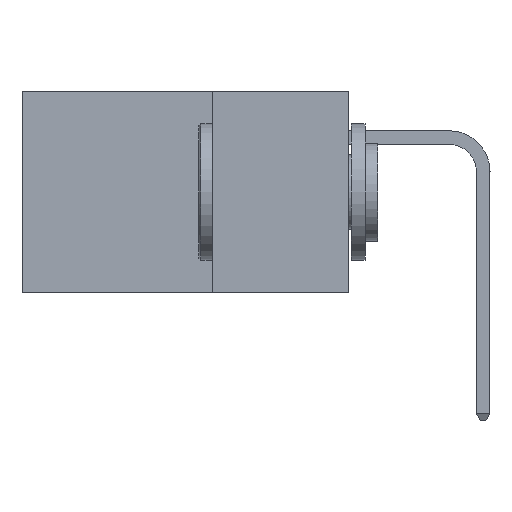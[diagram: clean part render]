
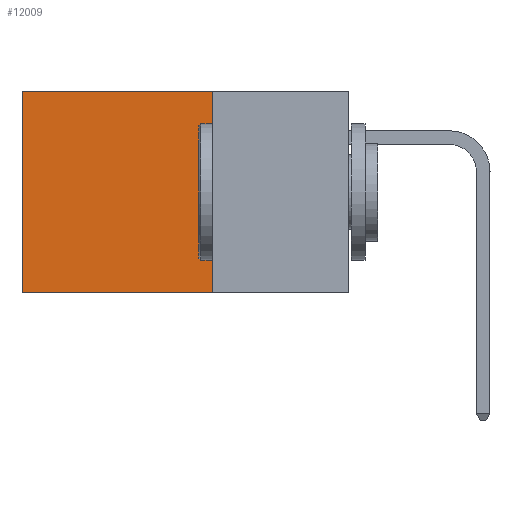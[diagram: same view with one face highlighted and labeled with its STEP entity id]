
A CAD part, left-side view. The second image highlights one B-rep face of the part: STEP entity #12009.
In plain terms, the highlighted planar face has unit normal (-1, 0, 0).
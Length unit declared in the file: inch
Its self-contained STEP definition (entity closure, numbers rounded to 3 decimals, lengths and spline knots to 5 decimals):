
#144 = PLANE ( 'NONE',  #20492 ) ;
#1122 = CARTESIAN_POINT ( 'NONE',  ( 0.2875, 0.6, 0. ) ) ;
#1136 = LINE ( 'NONE', #16714, #17392 ) ;
#1546 = VERTEX_POINT ( 'NONE', #5032 ) ;
#2478 = CARTESIAN_POINT ( 'NONE',  ( 0.2875, 0.25, 0. ) ) ;
#2580 = EDGE_CURVE ( 'NONE', #22776, #1546, #17502, .T. ) ;
#2743 = DIRECTION ( 'NONE',  ( 0., 0., -1. ) ) ;
#3334 = VECTOR ( 'NONE', #19300, 39.37008 ) ;
#3573 = CARTESIAN_POINT ( 'NONE',  ( 0.2875, 0.6, -0.37 ) ) ;
#3622 = VERTEX_POINT ( 'NONE', #3573 ) ;
#5032 = CARTESIAN_POINT ( 'NONE',  ( 0.2875, 0.6, 0. ) ) ;
#7667 = LINE ( 'NONE', #15661, #23456 ) ;
#8978 = CARTESIAN_POINT ( 'NONE',  ( 0.2875, 0.25, 0. ) ) ;
#9780 = ORIENTED_EDGE ( 'NONE', *, *, #13392, .F. ) ;
#12009 = ADVANCED_FACE ( 'NONE', ( #12944 ), #144, .F. ) ;
#12671 = VECTOR ( 'NONE', #15563, 39.37008 ) ;
#12944 = FACE_OUTER_BOUND ( 'NONE', #19693, .T. ) ;
#13011 = CARTESIAN_POINT ( 'NONE',  ( 0.2875, 0.25, 0. ) ) ;
#13283 = CARTESIAN_POINT ( 'NONE',  ( 0.2875, 0.25, -0.37 ) ) ;
#13392 = EDGE_CURVE ( 'NONE', #13552, #3622, #1136, .T. ) ;
#13552 = VERTEX_POINT ( 'NONE', #13283 ) ;
#13673 = EDGE_CURVE ( 'NONE', #22776, #13552, #7667, .T. ) ;
#14781 = ORIENTED_EDGE ( 'NONE', *, *, #16775, .T. ) ;
#15563 = DIRECTION ( 'NONE',  ( 0., 1., 0. ) ) ;
#15661 = CARTESIAN_POINT ( 'NONE',  ( 0.2875, 0.25, 0. ) ) ;
#16714 = CARTESIAN_POINT ( 'NONE',  ( 0.2875, 0.25, -0.37 ) ) ;
#16775 = EDGE_CURVE ( 'NONE', #1546, #3622, #23654, .T. ) ;
#17392 = VECTOR ( 'NONE', #20325, 39.37008 ) ;
#17502 = LINE ( 'NONE', #2478, #12671 ) ;
#17533 = ORIENTED_EDGE ( 'NONE', *, *, #2580, .T. ) ;
#17984 = DIRECTION ( 'NONE',  ( 0., 0., -1. ) ) ;
#18344 = DIRECTION ( 'NONE',  ( 1., 0., 0. ) ) ;
#19300 = DIRECTION ( 'NONE',  ( 0., 0., -1. ) ) ;
#19693 = EDGE_LOOP ( 'NONE', ( #14781, #9780, #20884, #17533 ) ) ;
#20325 = DIRECTION ( 'NONE',  ( 0., 1., 0. ) ) ;
#20492 = AXIS2_PLACEMENT_3D ( 'NONE', #8978, #18344, #17984 ) ;
#20884 = ORIENTED_EDGE ( 'NONE', *, *, #13673, .F. ) ;
#22776 = VERTEX_POINT ( 'NONE', #13011 ) ;
#23456 = VECTOR ( 'NONE', #2743, 39.37008 ) ;
#23654 = LINE ( 'NONE', #1122, #3334 ) ;
